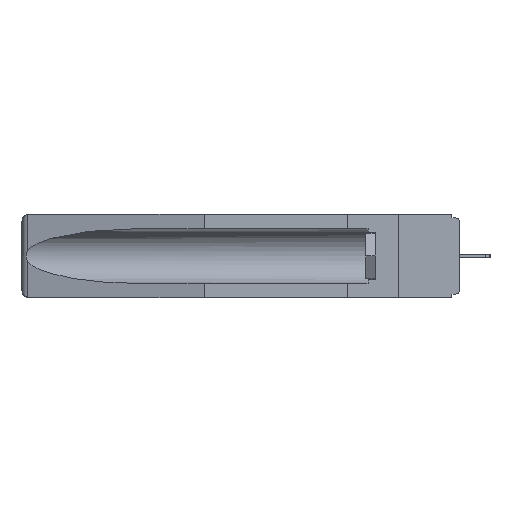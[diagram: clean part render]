
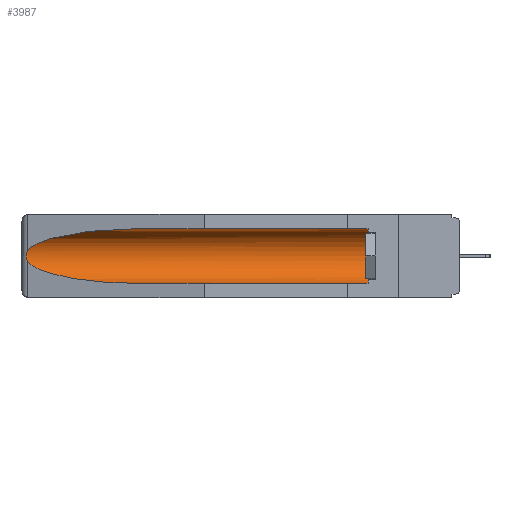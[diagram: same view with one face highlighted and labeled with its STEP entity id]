
A CAD part, left-side view. The second image highlights one B-rep face of the part: STEP entity #3987.
In plain terms, the highlighted cylindrical face has radius 2.857 mm (diameter 5.715 mm), a partial arc.
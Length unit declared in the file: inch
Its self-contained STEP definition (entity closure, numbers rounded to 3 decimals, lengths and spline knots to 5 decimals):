
#221 = ORIENTED_EDGE ( 'NONE', *, *, #20884, .T. ) ;
#827 = CARTESIAN_POINT ( 'NONE',  ( 0.26537, 1.52718, -0.14972 ) ) ;
#992 = CARTESIAN_POINT ( 'NONE',  ( 0.155, -0.30754, -0.1715 ) ) ;
#1390 = CIRCLE ( 'NONE', #5718, 0.1125 ) ;
#1707 = CARTESIAN_POINT ( 'NONE',  ( 0.155, -0.30754, -0.284 ) ) ;
#1742 = CARTESIAN_POINT ( 'NONE',  ( 0.155, 0.126, -0.059 ) ) ;
#2345 = CARTESIAN_POINT ( 'NONE',  ( 0.2675, 1.53308, -0.16763 ) ) ;
#2367 = CARTESIAN_POINT ( 'NONE',  ( 0.2673, 1.5327, -0.16383 ) ) ;
#2398 = CARTESIAN_POINT ( 'NONE',  ( 0.26537, 1.52718, -0.19328 ) ) ;
#2479 = CARTESIAN_POINT ( 'NONE',  ( 0.26654, 1.53092, -0.15636 ) ) ;
#2670 = EDGE_CURVE ( 'NONE', #9680, #24139, #13961, .T. ) ;
#2685 = CARTESIAN_POINT ( 'NONE',  ( 0.25451, 1.48313, -0.09465 ) ) ;
#2745 = ORIENTED_EDGE ( 'NONE', *, *, #14057, .F. ) ;
#3242 = EDGE_CURVE ( 'NONE', #8239, #10407, #19269, .T. ) ;
#3987 = ADVANCED_FACE ( 'NONE', ( #7377 ), #12027, .F. ) ;
#4419 = CARTESIAN_POINT ( 'NONE',  ( 0.26537, 1.52718, -0.14972 ) ) ;
#4781 = LINE ( 'NONE', #1707, #10067 ) ;
#5115 = CARTESIAN_POINT ( 'NONE',  ( 0.155, 1.07973, -0.284 ) ) ;
#5351 = VERTEX_POINT ( 'NONE', #11265 ) ;
#5416 = EDGE_CURVE ( 'NONE', #5351, #9680, #1390, .T. ) ;
#5548 = ORIENTED_EDGE ( 'NONE', *, *, #2670, .T. ) ;
#5718 = AXIS2_PLACEMENT_3D ( 'NONE', #19297, #7534, #21231 ) ;
#6606 = EDGE_CURVE ( 'NONE', #10407, #15245, #13214, .T. ) ;
#7099 = ORIENTED_EDGE ( 'NONE', *, *, #6606, .T. ) ;
#7123 = CARTESIAN_POINT ( 'NONE',  ( 0.26597, 1.5296, -0.19026 ) ) ;
#7377 = FACE_OUTER_BOUND ( 'NONE', #18059, .T. ) ;
#7534 = DIRECTION ( 'NONE',  ( 0., -1., 0. ) ) ;
#7552 = CARTESIAN_POINT ( 'NONE',  ( 0.2675, 1.53308, -0.17534 ) ) ;
#7601 = CARTESIAN_POINT ( 'NONE',  ( 0.26537, 1.52718, -0.19328 ) ) ;
#7976 =( BOUNDED_CURVE ( )  B_SPLINE_CURVE ( 3, ( #8589, #20348, #2685, #16514 ),
 .UNSPECIFIED., .F., .F. ) 
 B_SPLINE_CURVE_WITH_KNOTS ( ( 4, 4 ),
 ( 4.71239, 6.08839 ),
 .UNSPECIFIED. ) 
 CURVE ( )  GEOMETRIC_REPRESENTATION_ITEM ( )  RATIONAL_B_SPLINE_CURVE ( ( 1., 0.848, 0.848, 1. ) ) 
 REPRESENTATION_ITEM ( '' )  );
#8239 = VERTEX_POINT ( 'NONE', #4419 ) ;
#8589 = CARTESIAN_POINT ( 'NONE',  ( 0.155, 1.07973, -0.059 ) ) ;
#8618 = CARTESIAN_POINT ( 'NONE',  ( 0.26655, 1.53094, -0.18657 ) ) ;
#8644 = CARTESIAN_POINT ( 'NONE',  ( 0.2673, 1.53269, -0.17917 ) ) ;
#8902 = DIRECTION ( 'NONE',  ( 0., 1., 0. ) ) ;
#9262 = ORIENTED_EDGE ( 'NONE', *, *, #3242, .T. ) ;
#9680 = VERTEX_POINT ( 'NONE', #1742 ) ;
#9964 = CARTESIAN_POINT ( 'NONE',  ( 0.155, -0.30754, -0.059 ) ) ;
#10067 = VECTOR ( 'NONE', #13600, 39.37008 ) ;
#10401 = CARTESIAN_POINT ( 'NONE',  ( 0.26597, 1.52961, -0.15275 ) ) ;
#10407 = VERTEX_POINT ( 'NONE', #2398 ) ;
#11023 = CARTESIAN_POINT ( 'NONE',  ( 0.25451, 1.48313, -0.24835 ) ) ;
#11265 = CARTESIAN_POINT ( 'NONE',  ( 0.155, 0.126, -0.284 ) ) ;
#11395 = CARTESIAN_POINT ( 'NONE',  ( 0.155, 1.07973, -0.059 ) ) ;
#12027 = CYLINDRICAL_SURFACE ( 'NONE', #24444, 0.1125 ) ;
#13024 = CARTESIAN_POINT ( 'NONE',  ( 0.26537, 1.52718, -0.19328 ) ) ;
#13214 =( BOUNDED_CURVE ( )  B_SPLINE_CURVE ( 3, ( #13024, #11023, #16930, #5115 ),
 .UNSPECIFIED., .F., .F. ) 
 B_SPLINE_CURVE_WITH_KNOTS ( ( 4, 4 ),
 ( 0.1948, 1.5708 ),
 .UNSPECIFIED. ) 
 CURVE ( )  GEOMETRIC_REPRESENTATION_ITEM ( )  RATIONAL_B_SPLINE_CURVE ( ( 1., 0.848, 0.848, 1. ) ) 
 REPRESENTATION_ITEM ( '' )  );
#13341 = VECTOR ( 'NONE', #21990, 39.37008 ) ;
#13600 = DIRECTION ( 'NONE',  ( 0., 1., 0. ) ) ;
#13961 = LINE ( 'NONE', #9964, #13341 ) ;
#14057 = EDGE_CURVE ( 'NONE', #5351, #15245, #4781, .T. ) ;
#15245 = VERTEX_POINT ( 'NONE', #18762 ) ;
#15750 = ORIENTED_EDGE ( 'NONE', *, *, #5416, .T. ) ;
#16514 = CARTESIAN_POINT ( 'NONE',  ( 0.26537, 1.52718, -0.14972 ) ) ;
#16930 = CARTESIAN_POINT ( 'NONE',  ( 0.21114, 1.30732, -0.284 ) ) ;
#18059 = EDGE_LOOP ( 'NONE', ( #221, #9262, #7099, #2745, #15750, #5548 ) ) ;
#18762 = CARTESIAN_POINT ( 'NONE',  ( 0.155, 1.07973, -0.284 ) ) ;
#19269 = B_SPLINE_CURVE_WITH_KNOTS ( 'NONE', 3,
 ( #827, #10401, #2479, #2367, #2345, #7552, #8644, #8618, #7123, #7601 ),
 .UNSPECIFIED., .F., .F.,
 ( 4, 2, 2, 2, 4 ),
 ( 0., 0.00029, 0.00058, 0.00087, 0.00117 ),
 .UNSPECIFIED. ) ;
#19297 = CARTESIAN_POINT ( 'NONE',  ( 0.155, 0.126, -0.1715 ) ) ;
#20348 = CARTESIAN_POINT ( 'NONE',  ( 0.21114, 1.30732, -0.059 ) ) ;
#20884 = EDGE_CURVE ( 'NONE', #24139, #8239, #7976, .T. ) ;
#21231 = DIRECTION ( 'NONE',  ( 0., 0., 1. ) ) ;
#21990 = DIRECTION ( 'NONE',  ( 0., 1., 0. ) ) ;
#24139 = VERTEX_POINT ( 'NONE', #11395 ) ;
#24444 = AXIS2_PLACEMENT_3D ( 'NONE', #992, #8902, #24563 ) ;
#24563 = DIRECTION ( 'NONE',  ( 0., 0., 1. ) ) ;
